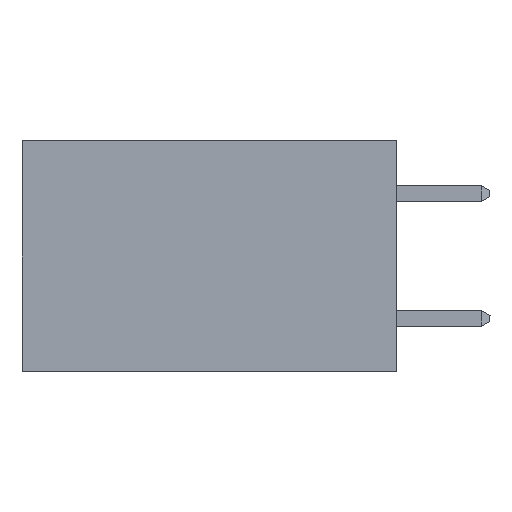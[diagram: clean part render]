
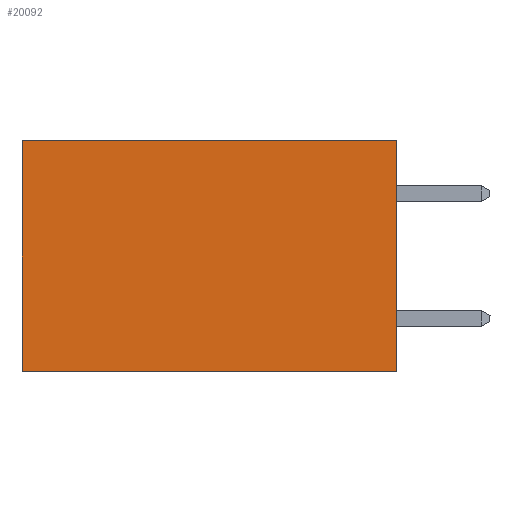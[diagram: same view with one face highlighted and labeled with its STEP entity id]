
A CAD part, left-side view. The second image highlights one B-rep face of the part: STEP entity #20092.
In plain terms, the highlighted planar face has unit normal (-1, 0, 0).
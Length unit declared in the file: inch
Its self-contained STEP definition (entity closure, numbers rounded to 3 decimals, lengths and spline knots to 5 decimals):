
#56 = CARTESIAN_POINT ( 'NONE',  ( 0.2615, 0., 0. ) ) ;
#422 = EDGE_CURVE ( 'NONE', #841, #6256, #19670, .T. ) ;
#841 = VERTEX_POINT ( 'NONE', #10116 ) ;
#1006 = DIRECTION ( 'NONE',  ( 0., 0., -1. ) ) ;
#1270 = CARTESIAN_POINT ( 'NONE',  ( 0.2615, 0., -0.37 ) ) ;
#2523 = LINE ( 'NONE', #21024, #15361 ) ;
#2983 = DIRECTION ( 'NONE',  ( 0., 0., -1. ) ) ;
#3184 = DIRECTION ( 'NONE',  ( 0., 1., 0. ) ) ;
#3559 = CARTESIAN_POINT ( 'NONE',  ( 0.2615, 0., 0. ) ) ;
#4363 = CARTESIAN_POINT ( 'NONE',  ( 0.2615, 0., -0.37 ) ) ;
#4727 = CARTESIAN_POINT ( 'NONE',  ( 0.2615, 0.6, -0.37 ) ) ;
#5079 = EDGE_LOOP ( 'NONE', ( #20583, #16895, #12629, #14969 ) ) ;
#5267 = DIRECTION ( 'NONE',  ( 0., 1., 0. ) ) ;
#5371 = EDGE_CURVE ( 'NONE', #11737, #841, #13550, .T. ) ;
#6256 = VERTEX_POINT ( 'NONE', #4727 ) ;
#6698 = FACE_OUTER_BOUND ( 'NONE', #5079, .T. ) ;
#7443 = EDGE_CURVE ( 'NONE', #11737, #21178, #8020, .T. ) ;
#8020 = LINE ( 'NONE', #3559, #20779 ) ;
#9210 = CARTESIAN_POINT ( 'NONE',  ( 0.2615, 0.6, 0. ) ) ;
#10116 = CARTESIAN_POINT ( 'NONE',  ( 0.2615, 0., -0.37 ) ) ;
#11737 = VERTEX_POINT ( 'NONE', #56 ) ;
#11838 = VECTOR ( 'NONE', #3184, 39.37008 ) ;
#12629 = ORIENTED_EDGE ( 'NONE', *, *, #5371, .F. ) ;
#12858 = EDGE_CURVE ( 'NONE', #21178, #6256, #2523, .T. ) ;
#13031 = DIRECTION ( 'NONE',  ( 1., 0., 0. ) ) ;
#13115 = DIRECTION ( 'NONE',  ( 0., 0., -1. ) ) ;
#13184 = CARTESIAN_POINT ( 'NONE',  ( 0.2615, 0., -0.37 ) ) ;
#13550 = LINE ( 'NONE', #13184, #14083 ) ;
#14083 = VECTOR ( 'NONE', #13115, 39.37008 ) ;
#14346 = AXIS2_PLACEMENT_3D ( 'NONE', #1270, #13031, #2983 ) ;
#14969 = ORIENTED_EDGE ( 'NONE', *, *, #7443, .T. ) ;
#15361 = VECTOR ( 'NONE', #1006, 39.37008 ) ;
#16895 = ORIENTED_EDGE ( 'NONE', *, *, #422, .F. ) ;
#19670 = LINE ( 'NONE', #4363, #11838 ) ;
#19672 = PLANE ( 'NONE',  #14346 ) ;
#20092 = ADVANCED_FACE ( 'NONE', ( #6698 ), #19672, .F. ) ;
#20583 = ORIENTED_EDGE ( 'NONE', *, *, #12858, .T. ) ;
#20779 = VECTOR ( 'NONE', #5267, 39.37008 ) ;
#21024 = CARTESIAN_POINT ( 'NONE',  ( 0.2615, 0.6, -0.37 ) ) ;
#21178 = VERTEX_POINT ( 'NONE', #9210 ) ;
